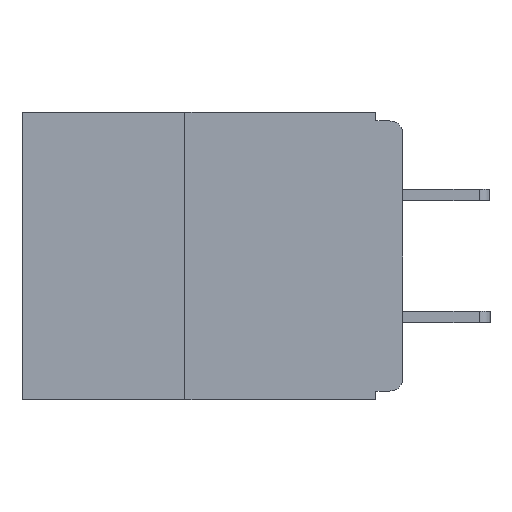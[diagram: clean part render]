
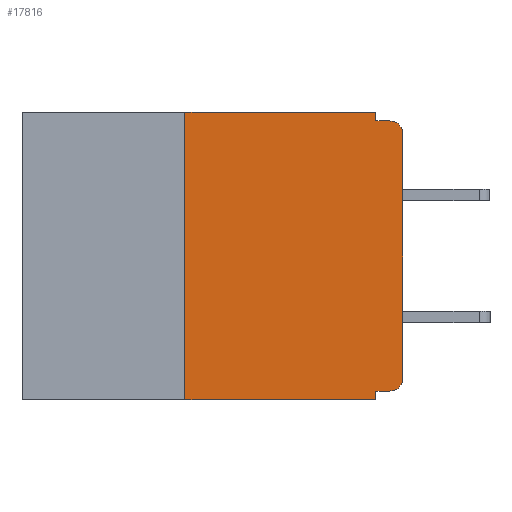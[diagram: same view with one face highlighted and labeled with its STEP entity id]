
A CAD part, left-side view. The second image highlights one B-rep face of the part: STEP entity #17816.
In plain terms, the highlighted planar face has unit normal (-1, 0, 0).
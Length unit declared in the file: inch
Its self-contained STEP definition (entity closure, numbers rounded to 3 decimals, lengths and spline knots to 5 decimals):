
#477 = ORIENTED_EDGE ( 'NONE', *, *, #30431, .T. ) ;
#1104 = VERTEX_POINT ( 'NONE', #19261 ) ;
#1455 = VECTOR ( 'NONE', #12010, 39.37008 ) ;
#1844 = VERTEX_POINT ( 'NONE', #20547 ) ;
#2181 = VERTEX_POINT ( 'NONE', #5809 ) ;
#2298 = CARTESIAN_POINT ( 'NONE',  ( 0., 0.031, 0. ) ) ;
#2380 = VECTOR ( 'NONE', #19283, 39.37008 ) ;
#3038 = EDGE_CURVE ( 'NONE', #2181, #9718, #8774, .T. ) ;
#3039 = VERTEX_POINT ( 'NONE', #19567 ) ;
#4596 = EDGE_CURVE ( 'NONE', #3039, #1844, #9045, .T. ) ;
#5809 = CARTESIAN_POINT ( 'NONE',  ( 0., 0.031, -0.01 ) ) ;
#6488 = CARTESIAN_POINT ( 'NONE',  ( 0., 0.25, -0.33 ) ) ;
#6670 = LINE ( 'NONE', #29037, #17945 ) ;
#6849 = CARTESIAN_POINT ( 'NONE',  ( 0., 0.25, -0.33 ) ) ;
#7358 = CIRCLE ( 'NONE', #29076, 0.015 ) ;
#7763 = CARTESIAN_POINT ( 'NONE',  ( 0., 0.437, -0.33 ) ) ;
#8032 = DIRECTION ( 'NONE',  ( 1., 0., 0. ) ) ;
#8467 = CARTESIAN_POINT ( 'NONE',  ( 0., 0., -0.32 ) ) ;
#8585 = LINE ( 'NONE', #2298, #1455 ) ;
#8747 = EDGE_CURVE ( 'NONE', #1844, #13304, #17970, .T. ) ;
#8774 = LINE ( 'NONE', #19423, #2380 ) ;
#9045 = LINE ( 'NONE', #8467, #27781 ) ;
#9587 = CARTESIAN_POINT ( 'NONE',  ( 0., 0.015, -0.305 ) ) ;
#9718 = VERTEX_POINT ( 'NONE', #29321 ) ;
#9921 = EDGE_CURVE ( 'NONE', #12821, #10232, #28763, .T. ) ;
#10116 = VECTOR ( 'NONE', #29977, 39.37008 ) ;
#10157 = EDGE_CURVE ( 'NONE', #12821, #13304, #23756, .T. ) ;
#10232 = VERTEX_POINT ( 'NONE', #26835 ) ;
#10478 = VECTOR ( 'NONE', #28809, 39.37008 ) ;
#10580 = ORIENTED_EDGE ( 'NONE', *, *, #4596, .F. ) ;
#10969 = ORIENTED_EDGE ( 'NONE', *, *, #19152, .T. ) ;
#11760 = VECTOR ( 'NONE', #25008, 39.37008 ) ;
#12010 = DIRECTION ( 'NONE',  ( 0., 0., -1. ) ) ;
#12042 = DIRECTION ( 'NONE',  ( 0., 0., -1. ) ) ;
#12110 = VERTEX_POINT ( 'NONE', #29589 ) ;
#12821 = VERTEX_POINT ( 'NONE', #6849 ) ;
#13015 = ORIENTED_EDGE ( 'NONE', *, *, #21563, .F. ) ;
#13304 = VERTEX_POINT ( 'NONE', #15288 ) ;
#13848 = DIRECTION ( 'NONE',  ( -1., 0., 0. ) ) ;
#14683 = ORIENTED_EDGE ( 'NONE', *, *, #9921, .F. ) ;
#15288 = CARTESIAN_POINT ( 'NONE',  ( 0., 0.031, -0.33 ) ) ;
#17064 = AXIS2_PLACEMENT_3D ( 'NONE', #27813, #13848, #30064 ) ;
#17511 = ORIENTED_EDGE ( 'NONE', *, *, #10157, .T. ) ;
#17816 = ADVANCED_FACE ( 'NONE', ( #20171 ), #22254, .F. ) ;
#17945 = VECTOR ( 'NONE', #18798, 39.37008 ) ;
#17970 = LINE ( 'NONE', #21341, #30179 ) ;
#18707 = ORIENTED_EDGE ( 'NONE', *, *, #25866, .F. ) ;
#18798 = DIRECTION ( 'NONE',  ( 0., 0., 1. ) ) ;
#19152 = EDGE_CURVE ( 'NONE', #3039, #12110, #7358, .T. ) ;
#19261 = CARTESIAN_POINT ( 'NONE',  ( 0., 0., -0.025 ) ) ;
#19283 = DIRECTION ( 'NONE',  ( 0., -1., 0. ) ) ;
#19423 = CARTESIAN_POINT ( 'NONE',  ( 0., 0., -0.01 ) ) ;
#19567 = CARTESIAN_POINT ( 'NONE',  ( 0., 0.015, -0.32 ) ) ;
#19585 = ORIENTED_EDGE ( 'NONE', *, *, #8747, .F. ) ;
#19695 = EDGE_CURVE ( 'NONE', #1104, #9718, #28650, .T. ) ;
#19954 = EDGE_LOOP ( 'NONE', ( #477, #26118, #29253, #13015, #18707, #14683, #17511, #19585, #10580, #10969 ) ) ;
#20171 = FACE_OUTER_BOUND ( 'NONE', #19954, .T. ) ;
#20422 = CARTESIAN_POINT ( 'NONE',  ( 0., 0.437, 0. ) ) ;
#20547 = CARTESIAN_POINT ( 'NONE',  ( 0., 0.031, -0.32 ) ) ;
#21341 = CARTESIAN_POINT ( 'NONE',  ( 0., 0.031, -0.33 ) ) ;
#21563 = EDGE_CURVE ( 'NONE', #22270, #2181, #8585, .T. ) ;
#21862 = AXIS2_PLACEMENT_3D ( 'NONE', #26803, #8032, #24600 ) ;
#22254 = PLANE ( 'NONE',  #21862 ) ;
#22270 = VERTEX_POINT ( 'NONE', #27336 ) ;
#22672 = DIRECTION ( 'NONE',  ( 0., 1., 0. ) ) ;
#23689 = DIRECTION ( 'NONE',  ( 0., 0., -1. ) ) ;
#23756 = LINE ( 'NONE', #7763, #10478 ) ;
#24600 = DIRECTION ( 'NONE',  ( 0., 0., -1. ) ) ;
#25008 = DIRECTION ( 'NONE',  ( 0., -1., 0. ) ) ;
#25866 = EDGE_CURVE ( 'NONE', #10232, #22270, #29594, .T. ) ;
#26077 = DIRECTION ( 'NONE',  ( -1., 0., 0. ) ) ;
#26118 = ORIENTED_EDGE ( 'NONE', *, *, #19695, .T. ) ;
#26803 = CARTESIAN_POINT ( 'NONE',  ( 0., 0.437, 0. ) ) ;
#26835 = CARTESIAN_POINT ( 'NONE',  ( 0., 0.25, 0. ) ) ;
#27336 = CARTESIAN_POINT ( 'NONE',  ( 0., 0.031, 0. ) ) ;
#27781 = VECTOR ( 'NONE', #22672, 39.37008 ) ;
#27813 = CARTESIAN_POINT ( 'NONE',  ( 0., 0.015, -0.025 ) ) ;
#28650 = CIRCLE ( 'NONE', #17064, 0.015 ) ;
#28763 = LINE ( 'NONE', #6488, #10116 ) ;
#28809 = DIRECTION ( 'NONE',  ( 0., -1., 0. ) ) ;
#29037 = CARTESIAN_POINT ( 'NONE',  ( 0., 0., 0. ) ) ;
#29076 = AXIS2_PLACEMENT_3D ( 'NONE', #9587, #26077, #12042 ) ;
#29253 = ORIENTED_EDGE ( 'NONE', *, *, #3038, .F. ) ;
#29321 = CARTESIAN_POINT ( 'NONE',  ( 0., 0.015, -0.01 ) ) ;
#29589 = CARTESIAN_POINT ( 'NONE',  ( 0., 0., -0.305 ) ) ;
#29594 = LINE ( 'NONE', #20422, #11760 ) ;
#29977 = DIRECTION ( 'NONE',  ( 0., 0., 1. ) ) ;
#30064 = DIRECTION ( 'NONE',  ( 0., 0., -1. ) ) ;
#30179 = VECTOR ( 'NONE', #23689, 39.37008 ) ;
#30431 = EDGE_CURVE ( 'NONE', #12110, #1104, #6670, .T. ) ;
